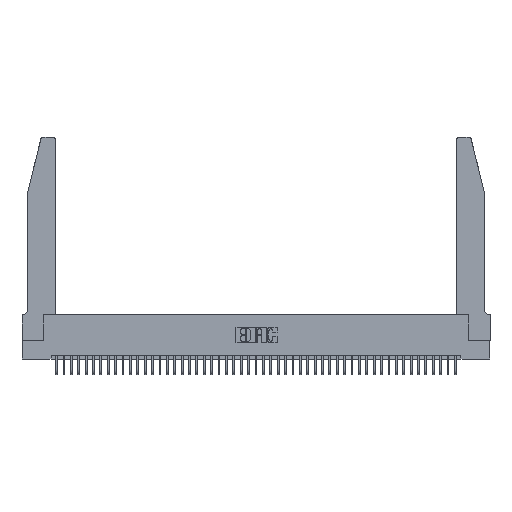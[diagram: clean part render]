
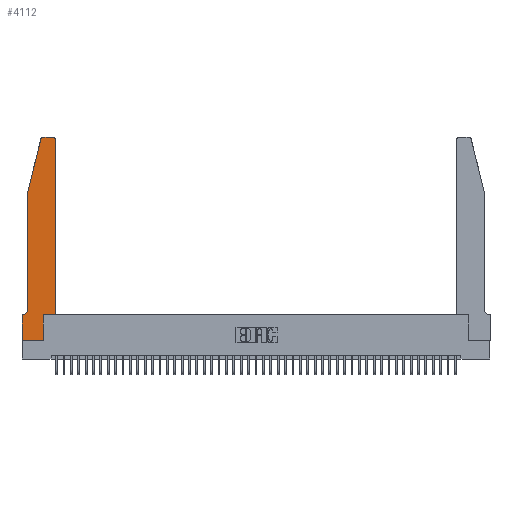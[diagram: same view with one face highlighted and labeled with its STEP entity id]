
A CAD part, top view. The second image highlights one B-rep face of the part: STEP entity #4112.
In plain terms, the highlighted planar face has unit normal (0, 0, 1).
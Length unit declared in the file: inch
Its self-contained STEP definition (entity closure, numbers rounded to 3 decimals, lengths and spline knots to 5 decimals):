
#800 = ORIENTED_EDGE ( 'NONE', *, *, #30918, .T. ) ;
#1379 = ORIENTED_EDGE ( 'NONE', *, *, #31925, .T. ) ;
#1502 = ORIENTED_EDGE ( 'NONE', *, *, #22042, .T. ) ;
#2519 = EDGE_CURVE ( 'NONE', #8407, #5817, #34613, .T. ) ;
#3063 = DIRECTION ( 'NONE',  ( 0., -1., 0. ) ) ;
#3406 = LINE ( 'NONE', #20316, #37464 ) ;
#3470 = EDGE_CURVE ( 'NONE', #22311, #28335, #3406, .T. ) ;
#4112 = ADVANCED_FACE ( 'NONE', ( #11410 ), #35054, .T. ) ;
#4418 = EDGE_CURVE ( 'NONE', #24645, #8407, #16619, .T. ) ;
#4553 = CARTESIAN_POINT ( 'NONE',  ( 0.0755, 2., 0.37 ) ) ;
#4879 = DIRECTION ( 'NONE',  ( 0., 1., 0. ) ) ;
#5447 = LINE ( 'NONE', #33277, #8909 ) ;
#5817 = VERTEX_POINT ( 'NONE', #42737 ) ;
#5908 = VERTEX_POINT ( 'NONE', #47609 ) ;
#6568 = LINE ( 'NONE', #31424, #44736 ) ;
#6921 = DIRECTION ( 'NONE',  ( 1., 0., 0. ) ) ;
#7632 = DIRECTION ( 'NONE',  ( 0., 0., 1. ) ) ;
#7761 = DIRECTION ( 'NONE',  ( -1., 0., 0. ) ) ;
#8407 = VERTEX_POINT ( 'NONE', #28422 ) ;
#8494 = CIRCLE ( 'NONE', #12329, 0.03 ) ;
#8650 = CARTESIAN_POINT ( 'NONE',  ( 0., 0.35, 0.37 ) ) ;
#8766 = CARTESIAN_POINT ( 'NONE',  ( 0.0055, 0.42, 0.37 ) ) ;
#8909 = VECTOR ( 'NONE', #41050, 39.37008 ) ;
#9659 = VECTOR ( 'NONE', #26842, 39.37008 ) ;
#10401 = ORIENTED_EDGE ( 'NONE', *, *, #39624, .T. ) ;
#11244 = VERTEX_POINT ( 'NONE', #33242 ) ;
#11410 = FACE_OUTER_BOUND ( 'NONE', #39213, .T. ) ;
#11555 = DIRECTION ( 'NONE',  ( 0., 1., 0. ) ) ;
#11812 = CARTESIAN_POINT ( 'NONE',  ( 0.4505, 0.35, 0.37 ) ) ;
#11845 = DIRECTION ( 'NONE',  ( -1., 0., 0. ) ) ;
#12329 = AXIS2_PLACEMENT_3D ( 'NONE', #37969, #19574, #15229 ) ;
#12401 = VERTEX_POINT ( 'NONE', #37690 ) ;
#12899 = DIRECTION ( 'NONE',  ( 1., 0., 0. ) ) ;
#13404 = LINE ( 'NONE', #46257, #29533 ) ;
#14112 = CARTESIAN_POINT ( 'NONE',  ( 0.25487, 2.72718, 0.37 ) ) ;
#14637 = AXIS2_PLACEMENT_3D ( 'NONE', #8650, #7632, #38177 ) ;
#14813 = CIRCLE ( 'NONE', #17115, 0.07 ) ;
#15186 = ORIENTED_EDGE ( 'NONE', *, *, #19569, .T. ) ;
#15229 = DIRECTION ( 'NONE',  ( 1., 0., 0. ) ) ;
#15765 = ORIENTED_EDGE ( 'NONE', *, *, #16277, .T. ) ;
#16277 = EDGE_CURVE ( 'NONE', #5817, #22311, #14813, .T. ) ;
#16495 = CARTESIAN_POINT ( 'NONE',  ( 0., 0.35, 0.37 ) ) ;
#16619 = LINE ( 'NONE', #4553, #9659 ) ;
#17056 = EDGE_CURVE ( 'NONE', #38872, #23579, #5447, .T. ) ;
#17115 = AXIS2_PLACEMENT_3D ( 'NONE', #8766, #41232, #11845 ) ;
#18554 = LINE ( 'NONE', #37215, #38774 ) ;
#19322 = DIRECTION ( 'NONE',  ( 0., -1., 0. ) ) ;
#19569 = EDGE_CURVE ( 'NONE', #28335, #22114, #27237, .T. ) ;
#19574 = DIRECTION ( 'NONE',  ( 0., 0., 1. ) ) ;
#20298 = EDGE_CURVE ( 'NONE', #5908, #43960, #29418, .T. ) ;
#20316 = CARTESIAN_POINT ( 'NONE',  ( 0.0755, 0.35, 0.37 ) ) ;
#21444 = CARTESIAN_POINT ( 'NONE',  ( 0.4205, 2.72, 0.37 ) ) ;
#21450 = CARTESIAN_POINT ( 'NONE',  ( 0., 0., 0.37 ) ) ;
#22042 = EDGE_CURVE ( 'NONE', #43960, #24645, #8494, .T. ) ;
#22114 = VERTEX_POINT ( 'NONE', #24955 ) ;
#22311 = VERTEX_POINT ( 'NONE', #33458 ) ;
#22319 = CARTESIAN_POINT ( 'NONE',  ( 0.2605, 2.75, 0.37 ) ) ;
#23579 = VERTEX_POINT ( 'NONE', #11812 ) ;
#24065 = ORIENTED_EDGE ( 'NONE', *, *, #17056, .T. ) ;
#24645 = VERTEX_POINT ( 'NONE', #14112 ) ;
#24891 = EDGE_CURVE ( 'NONE', #23579, #12401, #13404, .T. ) ;
#24955 = CARTESIAN_POINT ( 'NONE',  ( 0., 0., 0.37 ) ) ;
#25451 = VECTOR ( 'NONE', #7761, 39.37008 ) ;
#25600 = ORIENTED_EDGE ( 'NONE', *, *, #4418, .T. ) ;
#26842 = DIRECTION ( 'NONE',  ( -0.239, -0.971, 0. ) ) ;
#27121 = VECTOR ( 'NONE', #19322, 39.37008 ) ;
#27160 = CARTESIAN_POINT ( 'NONE',  ( 0.2865, 0.35, 0.37 ) ) ;
#27237 = LINE ( 'NONE', #21450, #44060 ) ;
#28335 = VERTEX_POINT ( 'NONE', #16495 ) ;
#28422 = CARTESIAN_POINT ( 'NONE',  ( 0.0755, 2., 0.37 ) ) ;
#28824 = DIRECTION ( 'NONE',  ( 0., 0., 1. ) ) ;
#29418 = LINE ( 'NONE', #22319, #25451 ) ;
#29533 = VECTOR ( 'NONE', #4879, 39.37008 ) ;
#30451 = AXIS2_PLACEMENT_3D ( 'NONE', #21444, #28824, #6921 ) ;
#30918 = EDGE_CURVE ( 'NONE', #11244, #38872, #18554, .T. ) ;
#31424 = CARTESIAN_POINT ( 'NONE',  ( 0., 0., 0.37 ) ) ;
#31925 = EDGE_CURVE ( 'NONE', #12401, #5908, #32271, .T. ) ;
#32271 = CIRCLE ( 'NONE', #30451, 0.03 ) ;
#32816 = ORIENTED_EDGE ( 'NONE', *, *, #3470, .T. ) ;
#33242 = CARTESIAN_POINT ( 'NONE',  ( 0.2865, 0., 0.37 ) ) ;
#33277 = CARTESIAN_POINT ( 'NONE',  ( 0.4505, 0.35, 0.37 ) ) ;
#33458 = CARTESIAN_POINT ( 'NONE',  ( 0.0055, 0.35, 0.37 ) ) ;
#34613 = LINE ( 'NONE', #41453, #27121 ) ;
#35054 = PLANE ( 'NONE',  #14637 ) ;
#37215 = CARTESIAN_POINT ( 'NONE',  ( 0.2865, 0.35, 0.37 ) ) ;
#37464 = VECTOR ( 'NONE', #42933, 39.37008 ) ;
#37690 = CARTESIAN_POINT ( 'NONE',  ( 0.4505, 2.72, 0.37 ) ) ;
#37969 = CARTESIAN_POINT ( 'NONE',  ( 0.284, 2.72, 0.37 ) ) ;
#38177 = DIRECTION ( 'NONE',  ( 1., 0., 0. ) ) ;
#38774 = VECTOR ( 'NONE', #11555, 39.37008 ) ;
#38872 = VERTEX_POINT ( 'NONE', #27160 ) ;
#39185 = CARTESIAN_POINT ( 'NONE',  ( 0.284, 2.75, 0.37 ) ) ;
#39213 = EDGE_LOOP ( 'NONE', ( #45446, #1502, #25600, #42376, #15765, #32816, #15186, #10401, #800, #24065, #44995, #1379 ) ) ;
#39624 = EDGE_CURVE ( 'NONE', #22114, #11244, #6568, .T. ) ;
#41050 = DIRECTION ( 'NONE',  ( 1., 0., 0. ) ) ;
#41232 = DIRECTION ( 'NONE',  ( 0., 0., -1. ) ) ;
#41453 = CARTESIAN_POINT ( 'NONE',  ( 0.0755, 2., 0.37 ) ) ;
#42376 = ORIENTED_EDGE ( 'NONE', *, *, #2519, .T. ) ;
#42737 = CARTESIAN_POINT ( 'NONE',  ( 0.0755, 0.42, 0.37 ) ) ;
#42933 = DIRECTION ( 'NONE',  ( -1., 0., 0. ) ) ;
#43960 = VERTEX_POINT ( 'NONE', #39185 ) ;
#44060 = VECTOR ( 'NONE', #3063, 39.37008 ) ;
#44736 = VECTOR ( 'NONE', #12899, 39.37008 ) ;
#44995 = ORIENTED_EDGE ( 'NONE', *, *, #24891, .T. ) ;
#45446 = ORIENTED_EDGE ( 'NONE', *, *, #20298, .T. ) ;
#46257 = CARTESIAN_POINT ( 'NONE',  ( 0.4505, 0.35, 0.37 ) ) ;
#47609 = CARTESIAN_POINT ( 'NONE',  ( 0.4205, 2.75, 0.37 ) ) ;
